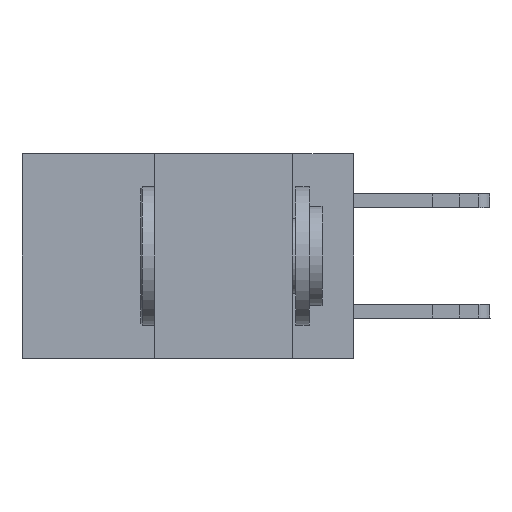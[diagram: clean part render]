
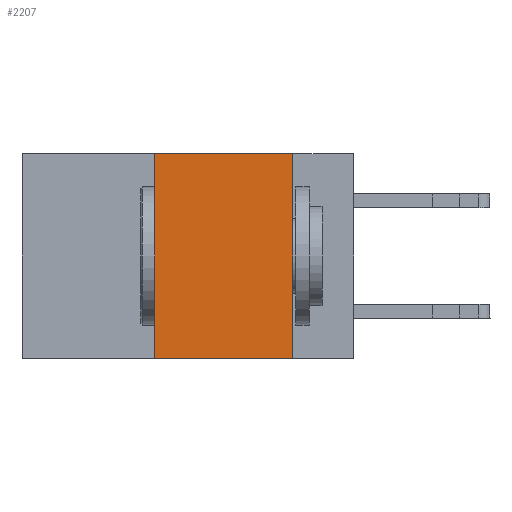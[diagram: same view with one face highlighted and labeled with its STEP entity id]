
A CAD part, left-side view. The second image highlights one B-rep face of the part: STEP entity #2207.
In plain terms, the highlighted planar face has unit normal (-1, 0, 0).
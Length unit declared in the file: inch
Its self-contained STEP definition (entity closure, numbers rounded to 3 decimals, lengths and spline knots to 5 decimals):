
#1926 = EDGE_CURVE ( 'NONE', #12329, #4917, #28109, .T. ) ;
#2207 = ADVANCED_FACE ( 'NONE', ( #13038 ), #23617, .F. ) ;
#3128 = CARTESIAN_POINT ( 'NONE',  ( 0., 0.36, 0. ) ) ;
#4917 = VERTEX_POINT ( 'NONE', #3128 ) ;
#6678 = ORIENTED_EDGE ( 'NONE', *, *, #10744, .F. ) ;
#7060 = CARTESIAN_POINT ( 'NONE',  ( 0., 0.6, 0. ) ) ;
#7238 = EDGE_CURVE ( 'NONE', #12329, #15471, #28825, .T. ) ;
#7455 = DIRECTION ( 'NONE',  ( 1., 0., 0. ) ) ;
#8720 = DIRECTION ( 'NONE',  ( 0., -1., 0. ) ) ;
#8832 = CARTESIAN_POINT ( 'NONE',  ( 0., 0.6, -0.37 ) ) ;
#9615 = ORIENTED_EDGE ( 'NONE', *, *, #22861, .F. ) ;
#10744 = EDGE_CURVE ( 'NONE', #16794, #15471, #21640, .T. ) ;
#11603 = VECTOR ( 'NONE', #8720, 39.37008 ) ;
#11706 = DIRECTION ( 'NONE',  ( 0., 0., -1. ) ) ;
#12030 = EDGE_LOOP ( 'NONE', ( #6678, #9615, #19416, #25657 ) ) ;
#12329 = VERTEX_POINT ( 'NONE', #20259 ) ;
#13038 = FACE_OUTER_BOUND ( 'NONE', #12030, .T. ) ;
#13182 = VECTOR ( 'NONE', #25386, 39.37008 ) ;
#14162 = CARTESIAN_POINT ( 'NONE',  ( 0., 0.36, 0. ) ) ;
#15471 = VERTEX_POINT ( 'NONE', #24370 ) ;
#16542 = DIRECTION ( 'NONE',  ( 0., 0., 1. ) ) ;
#16794 = VERTEX_POINT ( 'NONE', #22482 ) ;
#18295 = AXIS2_PLACEMENT_3D ( 'NONE', #7060, #7455, #11706 ) ;
#18700 = CARTESIAN_POINT ( 'NONE',  ( 0., 0.6, 0. ) ) ;
#19416 = ORIENTED_EDGE ( 'NONE', *, *, #1926, .F. ) ;
#20259 = CARTESIAN_POINT ( 'NONE',  ( 0., 0.36, -0.37 ) ) ;
#21640 = LINE ( 'NONE', #22957, #13182 ) ;
#22482 = CARTESIAN_POINT ( 'NONE',  ( 0., 0.11, 0. ) ) ;
#22861 = EDGE_CURVE ( 'NONE', #4917, #16794, #26869, .T. ) ;
#22957 = CARTESIAN_POINT ( 'NONE',  ( 0., 0.11, 0. ) ) ;
#23379 = VECTOR ( 'NONE', #16542, 39.37008 ) ;
#23617 = PLANE ( 'NONE',  #18295 ) ;
#24370 = CARTESIAN_POINT ( 'NONE',  ( 0., 0.11, -0.37 ) ) ;
#25386 = DIRECTION ( 'NONE',  ( 0., 0., -1. ) ) ;
#25406 = VECTOR ( 'NONE', #25740, 39.37008 ) ;
#25657 = ORIENTED_EDGE ( 'NONE', *, *, #7238, .T. ) ;
#25740 = DIRECTION ( 'NONE',  ( 0., -1., 0. ) ) ;
#26869 = LINE ( 'NONE', #18700, #25406 ) ;
#28109 = LINE ( 'NONE', #14162, #23379 ) ;
#28825 = LINE ( 'NONE', #8832, #11603 ) ;
